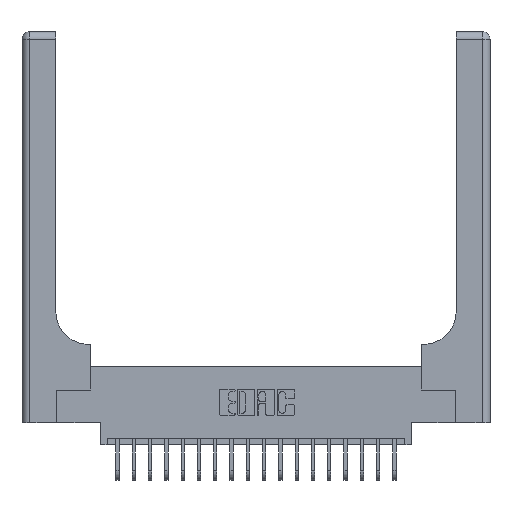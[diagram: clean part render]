
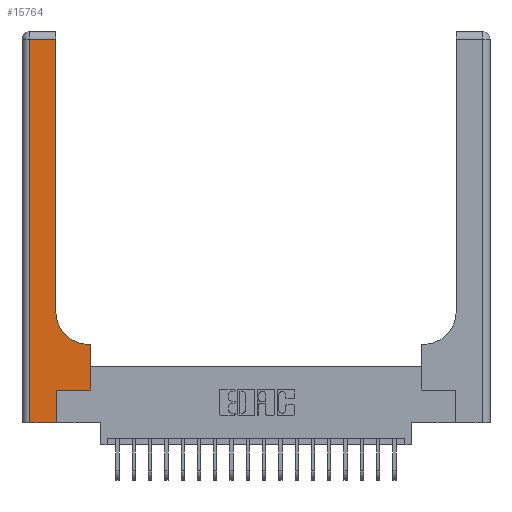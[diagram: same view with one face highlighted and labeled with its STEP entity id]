
A CAD part, top view. The second image highlights one B-rep face of the part: STEP entity #15764.
In plain terms, the highlighted planar face has unit normal (0, 0, 1).
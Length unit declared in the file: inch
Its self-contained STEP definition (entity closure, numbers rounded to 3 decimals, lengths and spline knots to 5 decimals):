
#68 = FACE_OUTER_BOUND ( 'NONE', #16805, .T. ) ;
#774 = CARTESIAN_POINT ( 'NONE',  ( 0.06, 3., 0.37 ) ) ;
#966 = DIRECTION ( 'NONE',  ( 1., 0., 0. ) ) ;
#1171 = AXIS2_PLACEMENT_3D ( 'NONE', #16869, #4378, #2846 ) ;
#1488 = CIRCLE ( 'NONE', #16206, 0.25 ) ;
#1670 = DIRECTION ( 'NONE',  ( -1., 0., 0. ) ) ;
#1824 = DIRECTION ( 'NONE',  ( 0., 1., 0. ) ) ;
#2132 = ORIENTED_EDGE ( 'NONE', *, *, #14345, .T. ) ;
#2134 = CARTESIAN_POINT ( 'NONE',  ( 0.51, 0.85, 0.37 ) ) ;
#2330 = LINE ( 'NONE', #10208, #11553 ) ;
#2509 = LINE ( 'NONE', #5470, #20006 ) ;
#2818 = CARTESIAN_POINT ( 'NONE',  ( 0.265, 0., 0.37 ) ) ;
#2846 = DIRECTION ( 'NONE',  ( -1., 0., 0. ) ) ;
#3125 = VERTEX_POINT ( 'NONE', #8941 ) ;
#3424 = VERTEX_POINT ( 'NONE', #4920 ) ;
#3962 = EDGE_CURVE ( 'NONE', #3424, #8472, #15757, .T. ) ;
#3969 = DIRECTION ( 'NONE',  ( -1., 0., 0. ) ) ;
#4144 = EDGE_CURVE ( 'NONE', #9643, #7733, #19521, .T. ) ;
#4259 = VERTEX_POINT ( 'NONE', #19935 ) ;
#4378 = DIRECTION ( 'NONE',  ( 0., 0., -1. ) ) ;
#4538 = LINE ( 'NONE', #2818, #5400 ) ;
#4652 = VERTEX_POINT ( 'NONE', #18670 ) ;
#4698 = CARTESIAN_POINT ( 'NONE',  ( 0.26, 3., 0.37 ) ) ;
#4920 = CARTESIAN_POINT ( 'NONE',  ( 0.26, 0.85, 0.37 ) ) ;
#5400 = VECTOR ( 'NONE', #5989, 39.37008 ) ;
#5470 = CARTESIAN_POINT ( 'NONE',  ( 0., 0., 0.37 ) ) ;
#5728 = VECTOR ( 'NONE', #1670, 39.37008 ) ;
#5989 = DIRECTION ( 'NONE',  ( 0., 1., 0. ) ) ;
#6056 = VERTEX_POINT ( 'NONE', #16110 ) ;
#6106 = DIRECTION ( 'NONE',  ( 0., 1., 0. ) ) ;
#7413 = VECTOR ( 'NONE', #1824, 39.37008 ) ;
#7630 = CARTESIAN_POINT ( 'NONE',  ( 0.528, 0.25, 0.37 ) ) ;
#7664 = VECTOR ( 'NONE', #16325, 39.37008 ) ;
#7733 = VERTEX_POINT ( 'NONE', #18212 ) ;
#8150 = DIRECTION ( 'NONE',  ( 0., 0., -1. ) ) ;
#8472 = VERTEX_POINT ( 'NONE', #18064 ) ;
#8666 = DIRECTION ( 'NONE',  ( 1., 0., 0. ) ) ;
#8941 = CARTESIAN_POINT ( 'NONE',  ( 0.265, 0., 0.37 ) ) ;
#9074 = ORIENTED_EDGE ( 'NONE', *, *, #12735, .T. ) ;
#9643 = VERTEX_POINT ( 'NONE', #11213 ) ;
#10208 = CARTESIAN_POINT ( 'NONE',  ( 0., 2.94, 0.37 ) ) ;
#10903 = ORIENTED_EDGE ( 'NONE', *, *, #11447, .T. ) ;
#11213 = CARTESIAN_POINT ( 'NONE',  ( 0.265, 0.25, 0.37 ) ) ;
#11291 = LINE ( 'NONE', #12522, #5728 ) ;
#11353 = ORIENTED_EDGE ( 'NONE', *, *, #15788, .T. ) ;
#11447 = EDGE_CURVE ( 'NONE', #4259, #3125, #2509, .T. ) ;
#11552 = DIRECTION ( 'NONE',  ( 1., 0., 0. ) ) ;
#11553 = VECTOR ( 'NONE', #3969, 39.37008 ) ;
#11725 = LINE ( 'NONE', #774, #7664 ) ;
#12289 = ORIENTED_EDGE ( 'NONE', *, *, #14555, .T. ) ;
#12522 = CARTESIAN_POINT ( 'NONE',  ( 0.26, 0.6, 0.37 ) ) ;
#12735 = EDGE_CURVE ( 'NONE', #8472, #6056, #2330, .T. ) ;
#13317 = VECTOR ( 'NONE', #8666, 39.37008 ) ;
#13978 = ORIENTED_EDGE ( 'NONE', *, *, #14575, .T. ) ;
#14345 = EDGE_CURVE ( 'NONE', #6056, #4259, #11725, .T. ) ;
#14555 = EDGE_CURVE ( 'NONE', #3125, #9643, #4538, .T. ) ;
#14575 = EDGE_CURVE ( 'NONE', #4652, #15353, #11291, .T. ) ;
#15330 = PLANE ( 'NONE',  #1171 ) ;
#15353 = VERTEX_POINT ( 'NONE', #18912 ) ;
#15489 = EDGE_CURVE ( 'NONE', #15353, #3424, #1488, .T. ) ;
#15757 = LINE ( 'NONE', #4698, #7413 ) ;
#15764 = ADVANCED_FACE ( 'NONE', ( #68 ), #15330, .F. ) ;
#15788 = EDGE_CURVE ( 'NONE', #7733, #4652, #17073, .T. ) ;
#16110 = CARTESIAN_POINT ( 'NONE',  ( 0.06, 2.94, 0.37 ) ) ;
#16206 = AXIS2_PLACEMENT_3D ( 'NONE', #2134, #8150, #11552 ) ;
#16325 = DIRECTION ( 'NONE',  ( 0., -1., 0. ) ) ;
#16467 = CARTESIAN_POINT ( 'NONE',  ( 0.265, 0.25, 0.37 ) ) ;
#16805 = EDGE_LOOP ( 'NONE', ( #17355, #9074, #2132, #10903, #12289, #18243, #11353, #13978, #17228 ) ) ;
#16869 = CARTESIAN_POINT ( 'NONE',  ( 0., 3., 0.37 ) ) ;
#17073 = LINE ( 'NONE', #7630, #20140 ) ;
#17228 = ORIENTED_EDGE ( 'NONE', *, *, #15489, .T. ) ;
#17355 = ORIENTED_EDGE ( 'NONE', *, *, #3962, .T. ) ;
#18064 = CARTESIAN_POINT ( 'NONE',  ( 0.26, 2.94, 0.37 ) ) ;
#18212 = CARTESIAN_POINT ( 'NONE',  ( 0.528, 0.25, 0.37 ) ) ;
#18243 = ORIENTED_EDGE ( 'NONE', *, *, #4144, .T. ) ;
#18670 = CARTESIAN_POINT ( 'NONE',  ( 0.528, 0.6, 0.37 ) ) ;
#18912 = CARTESIAN_POINT ( 'NONE',  ( 0.51, 0.6, 0.37 ) ) ;
#19521 = LINE ( 'NONE', #16467, #13317 ) ;
#19935 = CARTESIAN_POINT ( 'NONE',  ( 0.06, 0., 0.37 ) ) ;
#20006 = VECTOR ( 'NONE', #966, 39.37008 ) ;
#20140 = VECTOR ( 'NONE', #6106, 39.37008 ) ;
